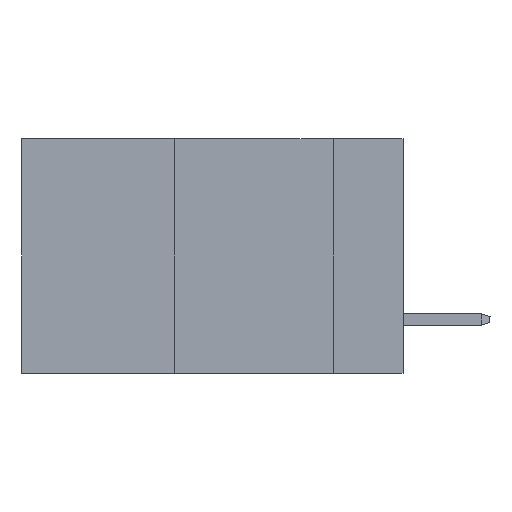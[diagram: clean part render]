
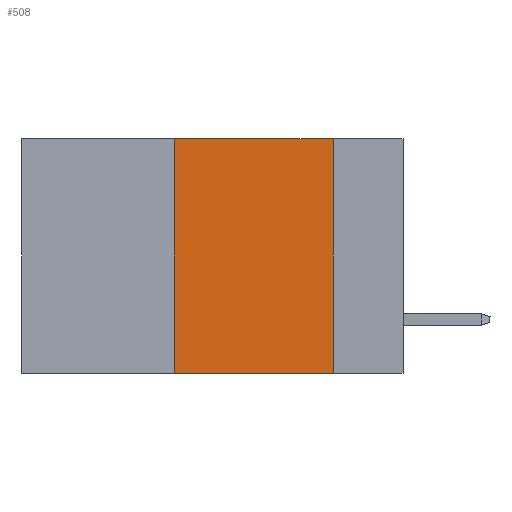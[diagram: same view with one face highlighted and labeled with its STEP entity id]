
A CAD part, left-side view. The second image highlights one B-rep face of the part: STEP entity #508.
In plain terms, the highlighted planar face has unit normal (-1, 0, 0).
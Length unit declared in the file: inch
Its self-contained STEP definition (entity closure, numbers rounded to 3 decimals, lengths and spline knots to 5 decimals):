
#508 = ADVANCED_FACE ( 'NONE', ( #17343 ), #9519, .F. ) ;
#1108 = CARTESIAN_POINT ( 'NONE',  ( 0., 0.11, 0. ) ) ;
#2667 = VECTOR ( 'NONE', #4105, 39.37008 ) ;
#2672 = ORIENTED_EDGE ( 'NONE', *, *, #20835, .F. ) ;
#4105 = DIRECTION ( 'NONE',  ( 0., -1., 0. ) ) ;
#5182 = EDGE_CURVE ( 'NONE', #8164, #15797, #8216, .T. ) ;
#5769 = CARTESIAN_POINT ( 'NONE',  ( 0., 0.36, 0. ) ) ;
#7718 = CARTESIAN_POINT ( 'NONE',  ( 0., 0.11, 0. ) ) ;
#8126 = DIRECTION ( 'NONE',  ( 0., 0., -1. ) ) ;
#8164 = VERTEX_POINT ( 'NONE', #18191 ) ;
#8216 = LINE ( 'NONE', #24166, #2667 ) ;
#8843 = DIRECTION ( 'NONE',  ( 0., -1., 0. ) ) ;
#9519 = PLANE ( 'NONE',  #16539 ) ;
#9652 = CARTESIAN_POINT ( 'NONE',  ( 0., 0.6, 0. ) ) ;
#11177 = VECTOR ( 'NONE', #8126, 39.37008 ) ;
#12342 = ORIENTED_EDGE ( 'NONE', *, *, #5182, .T. ) ;
#12658 = LINE ( 'NONE', #14643, #12868 ) ;
#12868 = VECTOR ( 'NONE', #18756, 39.37008 ) ;
#14030 = VECTOR ( 'NONE', #8843, 39.37008 ) ;
#14475 = ORIENTED_EDGE ( 'NONE', *, *, #17070, .F. ) ;
#14643 = CARTESIAN_POINT ( 'NONE',  ( 0., 0.36, 0. ) ) ;
#15797 = VERTEX_POINT ( 'NONE', #18907 ) ;
#16539 = AXIS2_PLACEMENT_3D ( 'NONE', #9652, #21455, #25594 ) ;
#17070 = EDGE_CURVE ( 'NONE', #19179, #20770, #23023, .T. ) ;
#17343 = FACE_OUTER_BOUND ( 'NONE', #20407, .T. ) ;
#17979 = ORIENTED_EDGE ( 'NONE', *, *, #19264, .F. ) ;
#18191 = CARTESIAN_POINT ( 'NONE',  ( 0., 0.36, -0.37 ) ) ;
#18756 = DIRECTION ( 'NONE',  ( 0., 0., 1. ) ) ;
#18907 = CARTESIAN_POINT ( 'NONE',  ( 0., 0.11, -0.37 ) ) ;
#19175 = CARTESIAN_POINT ( 'NONE',  ( 0., 0.6, 0. ) ) ;
#19179 = VERTEX_POINT ( 'NONE', #5769 ) ;
#19264 = EDGE_CURVE ( 'NONE', #8164, #19179, #12658, .T. ) ;
#20407 = EDGE_LOOP ( 'NONE', ( #2672, #14475, #17979, #12342 ) ) ;
#20770 = VERTEX_POINT ( 'NONE', #1108 ) ;
#20835 = EDGE_CURVE ( 'NONE', #20770, #15797, #24322, .T. ) ;
#21455 = DIRECTION ( 'NONE',  ( 1., 0., 0. ) ) ;
#23023 = LINE ( 'NONE', #19175, #14030 ) ;
#24166 = CARTESIAN_POINT ( 'NONE',  ( 0., 0.6, -0.37 ) ) ;
#24322 = LINE ( 'NONE', #7718, #11177 ) ;
#25594 = DIRECTION ( 'NONE',  ( 0., 0., -1. ) ) ;
